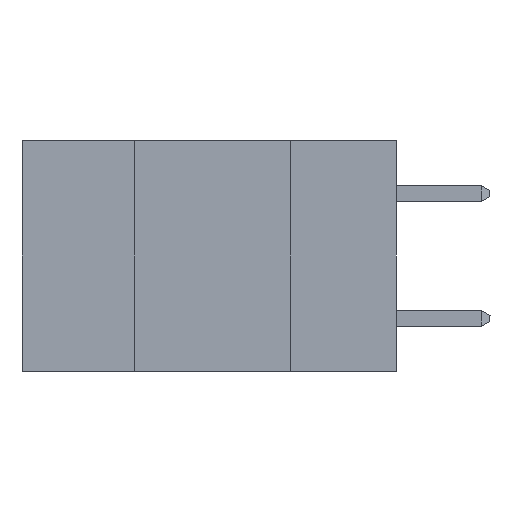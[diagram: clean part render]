
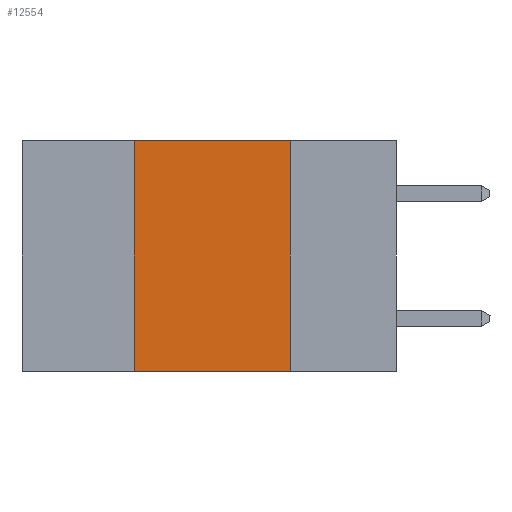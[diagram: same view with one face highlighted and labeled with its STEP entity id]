
A CAD part, left-side view. The second image highlights one B-rep face of the part: STEP entity #12554.
In plain terms, the highlighted planar face has unit normal (-1, 0, 0).
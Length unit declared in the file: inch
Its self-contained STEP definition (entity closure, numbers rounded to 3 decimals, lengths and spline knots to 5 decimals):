
#209 = DIRECTION ( 'NONE',  ( 0., 0., -1. ) ) ;
#518 = CARTESIAN_POINT ( 'NONE',  ( 0., 0.42, 0. ) ) ;
#973 = VERTEX_POINT ( 'NONE', #1030 ) ;
#1030 = CARTESIAN_POINT ( 'NONE',  ( 0., 0.17, 0. ) ) ;
#2106 = VERTEX_POINT ( 'NONE', #518 ) ;
#2303 = ORIENTED_EDGE ( 'NONE', *, *, #18333, .F. ) ;
#3955 = DIRECTION ( 'NONE',  ( 0., 0., -1. ) ) ;
#4822 = VECTOR ( 'NONE', #6259, 39.37008 ) ;
#5348 = FACE_OUTER_BOUND ( 'NONE', #6402, .T. ) ;
#6013 = CARTESIAN_POINT ( 'NONE',  ( 0., 0.42, 0. ) ) ;
#6259 = DIRECTION ( 'NONE',  ( 0., -1., 0. ) ) ;
#6402 = EDGE_LOOP ( 'NONE', ( #13567, #18862, #2303, #11178 ) ) ;
#6952 = LINE ( 'NONE', #16538, #4822 ) ;
#7154 = CARTESIAN_POINT ( 'NONE',  ( 0., 0.42, -0.37 ) ) ;
#8288 = LINE ( 'NONE', #17924, #16890 ) ;
#9893 = DIRECTION ( 'NONE',  ( 0., -1., 0. ) ) ;
#10587 = EDGE_CURVE ( 'NONE', #10824, #19120, #11009, .T. ) ;
#10762 = VECTOR ( 'NONE', #9893, 39.37008 ) ;
#10824 = VERTEX_POINT ( 'NONE', #7154 ) ;
#10870 = DIRECTION ( 'NONE',  ( 0., 0., 1. ) ) ;
#11009 = LINE ( 'NONE', #17013, #10762 ) ;
#11178 = ORIENTED_EDGE ( 'NONE', *, *, #10587, .T. ) ;
#11781 = EDGE_CURVE ( 'NONE', #973, #19120, #8288, .T. ) ;
#11984 = DIRECTION ( 'NONE',  ( 1., 0., 0. ) ) ;
#12554 = ADVANCED_FACE ( 'NONE', ( #5348 ), #16927, .F. ) ;
#12884 = AXIS2_PLACEMENT_3D ( 'NONE', #20637, #11984, #209 ) ;
#13162 = CARTESIAN_POINT ( 'NONE',  ( 0., 0.17, -0.37 ) ) ;
#13567 = ORIENTED_EDGE ( 'NONE', *, *, #11781, .F. ) ;
#16538 = CARTESIAN_POINT ( 'NONE',  ( 0., 0.6, 0. ) ) ;
#16890 = VECTOR ( 'NONE', #3955, 39.37008 ) ;
#16927 = PLANE ( 'NONE',  #12884 ) ;
#17013 = CARTESIAN_POINT ( 'NONE',  ( 0., 0.6, -0.37 ) ) ;
#17924 = CARTESIAN_POINT ( 'NONE',  ( 0., 0.17, 0. ) ) ;
#18034 = VECTOR ( 'NONE', #10870, 39.37008 ) ;
#18333 = EDGE_CURVE ( 'NONE', #10824, #2106, #21003, .T. ) ;
#18862 = ORIENTED_EDGE ( 'NONE', *, *, #19061, .F. ) ;
#19061 = EDGE_CURVE ( 'NONE', #2106, #973, #6952, .T. ) ;
#19120 = VERTEX_POINT ( 'NONE', #13162 ) ;
#20637 = CARTESIAN_POINT ( 'NONE',  ( 0., 0.6, 0. ) ) ;
#21003 = LINE ( 'NONE', #6013, #18034 ) ;
